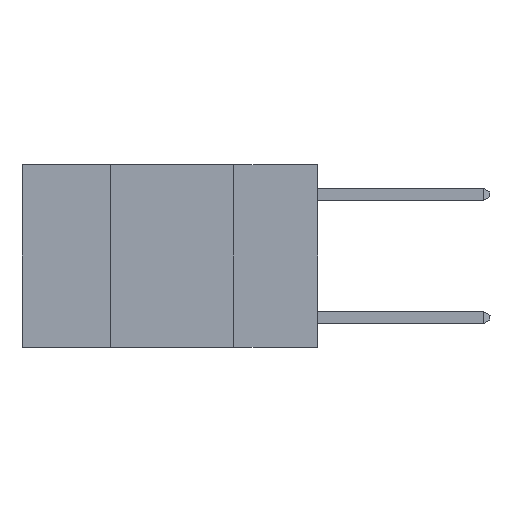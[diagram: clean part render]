
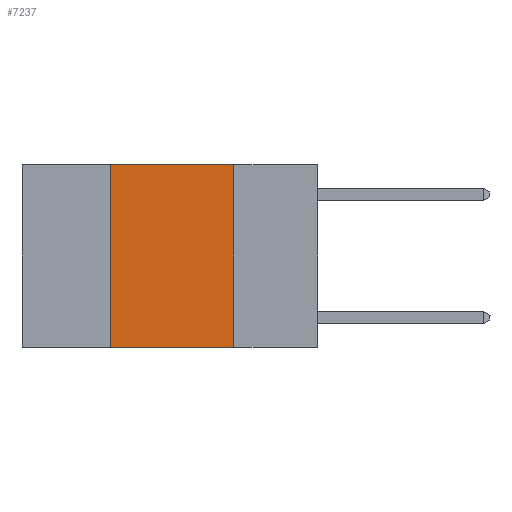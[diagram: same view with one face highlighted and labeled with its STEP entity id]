
A CAD part, left-side view. The second image highlights one B-rep face of the part: STEP entity #7237.
In plain terms, the highlighted planar face has unit normal (-1, 0, 0).
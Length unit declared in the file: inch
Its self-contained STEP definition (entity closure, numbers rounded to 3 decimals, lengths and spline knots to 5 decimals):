
#43 = DIRECTION ( 'NONE',  ( 0., -1., 0. ) ) ;
#623 = CARTESIAN_POINT ( 'NONE',  ( 0., 0.42, -0.37 ) ) ;
#3021 = DIRECTION ( 'NONE',  ( 0., 0., 1. ) ) ;
#3597 = EDGE_CURVE ( 'NONE', #16214, #24075, #5857, .T. ) ;
#3888 = CARTESIAN_POINT ( 'NONE',  ( 0., 0.6, 0. ) ) ;
#4456 = DIRECTION ( 'NONE',  ( 0., -1., 0. ) ) ;
#4815 = CARTESIAN_POINT ( 'NONE',  ( 0., 0.17, -0.37 ) ) ;
#5672 = VECTOR ( 'NONE', #3021, 39.37008 ) ;
#5857 = LINE ( 'NONE', #15378, #27069 ) ;
#7237 = ADVANCED_FACE ( 'NONE', ( #10471 ), #25313, .F. ) ;
#8664 = LINE ( 'NONE', #18639, #20069 ) ;
#8796 = CARTESIAN_POINT ( 'NONE',  ( 0., 0.17, 0. ) ) ;
#9890 = AXIS2_PLACEMENT_3D ( 'NONE', #3888, #27344, #15029 ) ;
#10471 = FACE_OUTER_BOUND ( 'NONE', #11371, .T. ) ;
#11371 = EDGE_LOOP ( 'NONE', ( #14768, #15115, #15462, #15498 ) ) ;
#14768 = ORIENTED_EDGE ( 'NONE', *, *, #27142, .F. ) ;
#15029 = DIRECTION ( 'NONE',  ( 0., 0., -1. ) ) ;
#15115 = ORIENTED_EDGE ( 'NONE', *, *, #3597, .F. ) ;
#15285 = VERTEX_POINT ( 'NONE', #623 ) ;
#15378 = CARTESIAN_POINT ( 'NONE',  ( 0., 0.6, 0. ) ) ;
#15462 = ORIENTED_EDGE ( 'NONE', *, *, #24430, .F. ) ;
#15498 = ORIENTED_EDGE ( 'NONE', *, *, #20316, .T. ) ;
#16214 = VERTEX_POINT ( 'NONE', #18132 ) ;
#18132 = CARTESIAN_POINT ( 'NONE',  ( 0., 0.42, 0. ) ) ;
#18299 = CARTESIAN_POINT ( 'NONE',  ( 0., 0.42, 0. ) ) ;
#18639 = CARTESIAN_POINT ( 'NONE',  ( 0., 0.17, 0. ) ) ;
#20069 = VECTOR ( 'NONE', #22787, 39.37008 ) ;
#20316 = EDGE_CURVE ( 'NONE', #15285, #21414, #22603, .T. ) ;
#21414 = VERTEX_POINT ( 'NONE', #4815 ) ;
#21702 = CARTESIAN_POINT ( 'NONE',  ( 0., 0.6, -0.37 ) ) ;
#22603 = LINE ( 'NONE', #21702, #23231 ) ;
#22787 = DIRECTION ( 'NONE',  ( 0., 0., -1. ) ) ;
#23231 = VECTOR ( 'NONE', #4456, 39.37008 ) ;
#24075 = VERTEX_POINT ( 'NONE', #8796 ) ;
#24430 = EDGE_CURVE ( 'NONE', #15285, #16214, #27543, .T. ) ;
#25313 = PLANE ( 'NONE',  #9890 ) ;
#27069 = VECTOR ( 'NONE', #43, 39.37008 ) ;
#27142 = EDGE_CURVE ( 'NONE', #24075, #21414, #8664, .T. ) ;
#27344 = DIRECTION ( 'NONE',  ( 1., 0., 0. ) ) ;
#27543 = LINE ( 'NONE', #18299, #5672 ) ;
